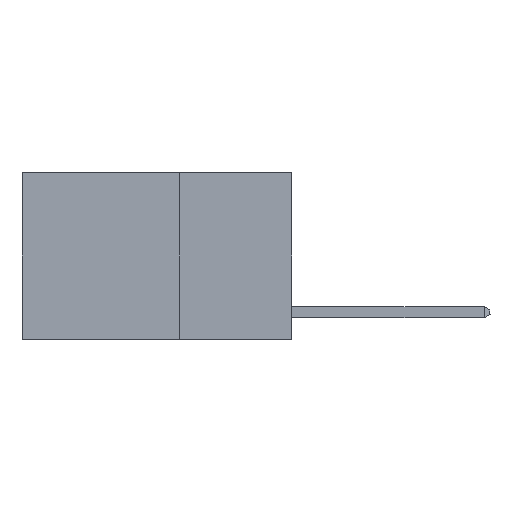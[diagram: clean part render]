
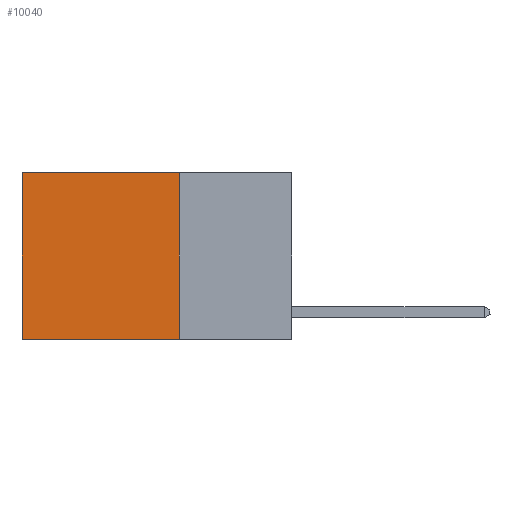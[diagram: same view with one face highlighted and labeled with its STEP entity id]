
A CAD part, left-side view. The second image highlights one B-rep face of the part: STEP entity #10040.
In plain terms, the highlighted planar face has unit normal (-1, 0, 0).
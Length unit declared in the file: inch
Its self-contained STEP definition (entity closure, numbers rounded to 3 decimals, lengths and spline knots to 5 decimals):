
#168 = ORIENTED_EDGE ( 'NONE', *, *, #10361, .T. ) ;
#238 = LINE ( 'NONE', #4926, #7633 ) ;
#428 = DIRECTION ( 'NONE',  ( 0., 0., -1. ) ) ;
#577 = VECTOR ( 'NONE', #11371, 39.37008 ) ;
#643 = EDGE_CURVE ( 'NONE', #7035, #11557, #238, .T. ) ;
#671 = ORIENTED_EDGE ( 'NONE', *, *, #643, .F. ) ;
#734 = CARTESIAN_POINT ( 'NONE',  ( 0.2625, 0.25, -0.37 ) ) ;
#969 = LINE ( 'NONE', #2113, #577 ) ;
#973 = CARTESIAN_POINT ( 'NONE',  ( 0.2625, 0.25, 0. ) ) ;
#1127 = CARTESIAN_POINT ( 'NONE',  ( 0.2625, 0.25, 0. ) ) ;
#1586 = LINE ( 'NONE', #14144, #7267 ) ;
#1749 = CARTESIAN_POINT ( 'NONE',  ( 0.2625, 0.6, -0.37 ) ) ;
#2113 = CARTESIAN_POINT ( 'NONE',  ( 0.2625, 0.25, 0. ) ) ;
#4391 = EDGE_LOOP ( 'NONE', ( #6803, #671, #4895, #168 ) ) ;
#4895 = ORIENTED_EDGE ( 'NONE', *, *, #6662, .F. ) ;
#4926 = CARTESIAN_POINT ( 'NONE',  ( 0.2625, 0.25, -0.37 ) ) ;
#5802 = LINE ( 'NONE', #1127, #7493 ) ;
#6662 = EDGE_CURVE ( 'NONE', #7935, #7035, #969, .T. ) ;
#6803 = ORIENTED_EDGE ( 'NONE', *, *, #11803, .T. ) ;
#6951 = VERTEX_POINT ( 'NONE', #13163 ) ;
#7035 = VERTEX_POINT ( 'NONE', #734 ) ;
#7074 = DIRECTION ( 'NONE',  ( 0., 0., -1. ) ) ;
#7267 = VECTOR ( 'NONE', #7074, 39.37008 ) ;
#7493 = VECTOR ( 'NONE', #11377, 39.37008 ) ;
#7633 = VECTOR ( 'NONE', #10721, 39.37008 ) ;
#7935 = VERTEX_POINT ( 'NONE', #973 ) ;
#8934 = AXIS2_PLACEMENT_3D ( 'NONE', #14503, #12025, #428 ) ;
#10040 = ADVANCED_FACE ( 'NONE', ( #13372 ), #11050, .F. ) ;
#10361 = EDGE_CURVE ( 'NONE', #7935, #6951, #5802, .T. ) ;
#10721 = DIRECTION ( 'NONE',  ( 0., 1., 0. ) ) ;
#11050 = PLANE ( 'NONE',  #8934 ) ;
#11371 = DIRECTION ( 'NONE',  ( 0., 0., -1. ) ) ;
#11377 = DIRECTION ( 'NONE',  ( 0., 1., 0. ) ) ;
#11557 = VERTEX_POINT ( 'NONE', #1749 ) ;
#11803 = EDGE_CURVE ( 'NONE', #6951, #11557, #1586, .T. ) ;
#12025 = DIRECTION ( 'NONE',  ( 1., 0., 0. ) ) ;
#13163 = CARTESIAN_POINT ( 'NONE',  ( 0.2625, 0.6, 0. ) ) ;
#13372 = FACE_OUTER_BOUND ( 'NONE', #4391, .T. ) ;
#14144 = CARTESIAN_POINT ( 'NONE',  ( 0.2625, 0.6, 0. ) ) ;
#14503 = CARTESIAN_POINT ( 'NONE',  ( 0.2625, 0.25, 0. ) ) ;
